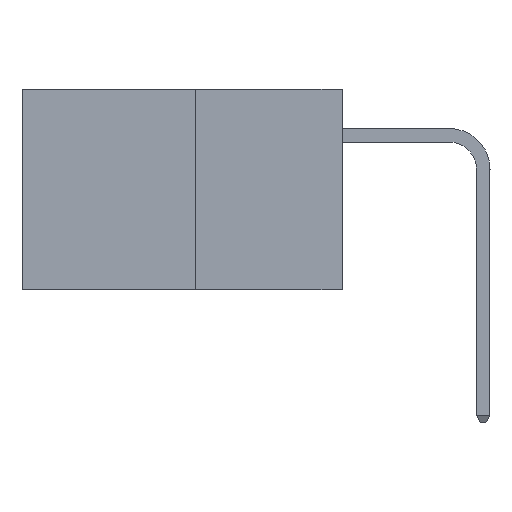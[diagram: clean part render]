
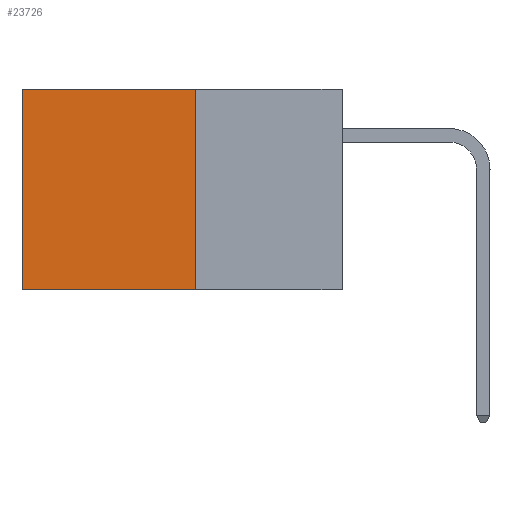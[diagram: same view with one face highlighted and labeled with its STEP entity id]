
A CAD part, left-side view. The second image highlights one B-rep face of the part: STEP entity #23726.
In plain terms, the highlighted planar face has unit normal (-1, 0, 0).
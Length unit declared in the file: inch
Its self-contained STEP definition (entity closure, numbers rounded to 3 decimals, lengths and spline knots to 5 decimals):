
#863 = VECTOR ( 'NONE', #2775, 39.37008 ) ;
#1375 = EDGE_LOOP ( 'NONE', ( #13014, #8400, #13331, #9810 ) ) ;
#2088 = CARTESIAN_POINT ( 'NONE',  ( 0.277, 0.27, -0.37 ) ) ;
#2775 = DIRECTION ( 'NONE',  ( 0., 1., 0. ) ) ;
#2858 = CARTESIAN_POINT ( 'NONE',  ( 0.277, 0.27, -0.37 ) ) ;
#4326 = CARTESIAN_POINT ( 'NONE',  ( 0.277, 0.27, -0.37 ) ) ;
#4448 = VERTEX_POINT ( 'NONE', #9783 ) ;
#4694 = VERTEX_POINT ( 'NONE', #6750 ) ;
#5053 = EDGE_CURVE ( 'NONE', #11566, #4694, #20690, .T. ) ;
#6328 = EDGE_CURVE ( 'NONE', #6600, #11566, #21554, .T. ) ;
#6600 = VERTEX_POINT ( 'NONE', #16300 ) ;
#6750 = CARTESIAN_POINT ( 'NONE',  ( 0.277, 0.59, -0.37 ) ) ;
#7362 = VECTOR ( 'NONE', #11727, 39.37008 ) ;
#7987 = LINE ( 'NONE', #9785, #7362 ) ;
#8400 = ORIENTED_EDGE ( 'NONE', *, *, #5053, .F. ) ;
#8410 = EDGE_CURVE ( 'NONE', #6600, #4448, #8570, .T. ) ;
#8554 = FACE_OUTER_BOUND ( 'NONE', #1375, .T. ) ;
#8570 = LINE ( 'NONE', #20958, #10373 ) ;
#9489 = DIRECTION ( 'NONE',  ( 0., 1., 0. ) ) ;
#9783 = CARTESIAN_POINT ( 'NONE',  ( 0.277, 0.59, 0. ) ) ;
#9785 = CARTESIAN_POINT ( 'NONE',  ( 0.277, 0.59, -0.37 ) ) ;
#9796 = CARTESIAN_POINT ( 'NONE',  ( 0.277, 0.27, -0.37 ) ) ;
#9810 = ORIENTED_EDGE ( 'NONE', *, *, #8410, .T. ) ;
#10373 = VECTOR ( 'NONE', #9489, 39.37008 ) ;
#11566 = VERTEX_POINT ( 'NONE', #9796 ) ;
#11700 = DIRECTION ( 'NONE',  ( 0., 0., -1. ) ) ;
#11727 = DIRECTION ( 'NONE',  ( 0., 0., -1. ) ) ;
#12094 = DIRECTION ( 'NONE',  ( 0., 0., -1. ) ) ;
#13014 = ORIENTED_EDGE ( 'NONE', *, *, #17767, .T. ) ;
#13331 = ORIENTED_EDGE ( 'NONE', *, *, #6328, .F. ) ;
#16300 = CARTESIAN_POINT ( 'NONE',  ( 0.277, 0.27, 0. ) ) ;
#17767 = EDGE_CURVE ( 'NONE', #4448, #4694, #7987, .T. ) ;
#17984 = AXIS2_PLACEMENT_3D ( 'NONE', #4326, #23542, #12094 ) ;
#20690 = LINE ( 'NONE', #2858, #863 ) ;
#20950 = VECTOR ( 'NONE', #11700, 39.37008 ) ;
#20958 = CARTESIAN_POINT ( 'NONE',  ( 0.277, 0.27, 0. ) ) ;
#21554 = LINE ( 'NONE', #2088, #20950 ) ;
#21617 = PLANE ( 'NONE',  #17984 ) ;
#23542 = DIRECTION ( 'NONE',  ( 1., 0., 0. ) ) ;
#23726 = ADVANCED_FACE ( 'NONE', ( #8554 ), #21617, .F. ) ;
